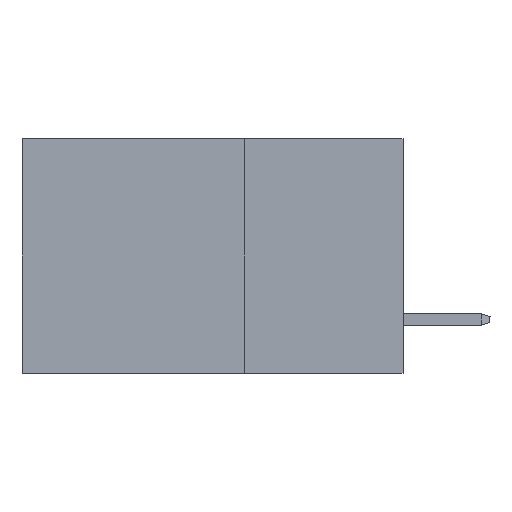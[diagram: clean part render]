
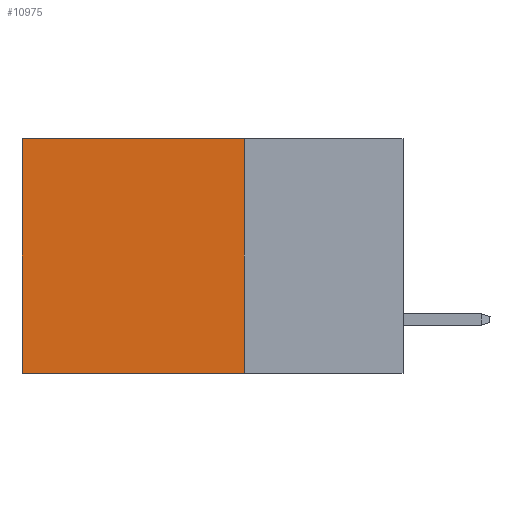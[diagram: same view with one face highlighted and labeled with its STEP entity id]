
A CAD part, left-side view. The second image highlights one B-rep face of the part: STEP entity #10975.
In plain terms, the highlighted planar face has unit normal (-1, 0, 0).
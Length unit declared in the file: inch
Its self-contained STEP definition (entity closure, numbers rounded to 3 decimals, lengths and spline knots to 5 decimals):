
#288 = LINE ( 'NONE', #14229, #12337 ) ;
#493 = AXIS2_PLACEMENT_3D ( 'NONE', #20267, #9228, #1410 ) ;
#652 = DIRECTION ( 'NONE',  ( 0., 0., -1. ) ) ;
#791 = EDGE_CURVE ( 'NONE', #18594, #16558, #288, .T. ) ;
#1067 = EDGE_LOOP ( 'NONE', ( #5371, #4088, #5901, #4847 ) ) ;
#1410 = DIRECTION ( 'NONE',  ( 0., 0., -1. ) ) ;
#1474 = CARTESIAN_POINT ( 'NONE',  ( 0.2875, 0.25, -0.37 ) ) ;
#2542 = VECTOR ( 'NONE', #19704, 39.37008 ) ;
#3211 = CARTESIAN_POINT ( 'NONE',  ( 0.2875, 0.6, -0.37 ) ) ;
#4088 = ORIENTED_EDGE ( 'NONE', *, *, #10537, .F. ) ;
#4847 = ORIENTED_EDGE ( 'NONE', *, *, #5748, .T. ) ;
#5371 = ORIENTED_EDGE ( 'NONE', *, *, #791, .T. ) ;
#5748 = EDGE_CURVE ( 'NONE', #11448, #18594, #15230, .T. ) ;
#5901 = ORIENTED_EDGE ( 'NONE', *, *, #19520, .F. ) ;
#7788 = VERTEX_POINT ( 'NONE', #1474 ) ;
#8547 = CARTESIAN_POINT ( 'NONE',  ( 0.2875, 0.25, 0. ) ) ;
#9228 = DIRECTION ( 'NONE',  ( 1., 0., 0. ) ) ;
#9898 = LINE ( 'NONE', #8547, #17374 ) ;
#10279 = DIRECTION ( 'NONE',  ( 0., 1., 0. ) ) ;
#10329 = CARTESIAN_POINT ( 'NONE',  ( 0.2875, 0.25, 0. ) ) ;
#10537 = EDGE_CURVE ( 'NONE', #7788, #16558, #12048, .T. ) ;
#10975 = ADVANCED_FACE ( 'NONE', ( #15665 ), #20457, .F. ) ;
#11448 = VERTEX_POINT ( 'NONE', #12474 ) ;
#11882 = CARTESIAN_POINT ( 'NONE',  ( 0.2875, 0.6, 0. ) ) ;
#12048 = LINE ( 'NONE', #20080, #18796 ) ;
#12337 = VECTOR ( 'NONE', #14420, 39.37008 ) ;
#12474 = CARTESIAN_POINT ( 'NONE',  ( 0.2875, 0.25, 0. ) ) ;
#14229 = CARTESIAN_POINT ( 'NONE',  ( 0.2875, 0.6, 0. ) ) ;
#14420 = DIRECTION ( 'NONE',  ( 0., 0., -1. ) ) ;
#15230 = LINE ( 'NONE', #10329, #2542 ) ;
#15665 = FACE_OUTER_BOUND ( 'NONE', #1067, .T. ) ;
#16558 = VERTEX_POINT ( 'NONE', #3211 ) ;
#17374 = VECTOR ( 'NONE', #652, 39.37008 ) ;
#18594 = VERTEX_POINT ( 'NONE', #11882 ) ;
#18796 = VECTOR ( 'NONE', #10279, 39.37008 ) ;
#19520 = EDGE_CURVE ( 'NONE', #11448, #7788, #9898, .T. ) ;
#19704 = DIRECTION ( 'NONE',  ( 0., 1., 0. ) ) ;
#20080 = CARTESIAN_POINT ( 'NONE',  ( 0.2875, 0.25, -0.37 ) ) ;
#20267 = CARTESIAN_POINT ( 'NONE',  ( 0.2875, 0.25, 0. ) ) ;
#20457 = PLANE ( 'NONE',  #493 ) ;
